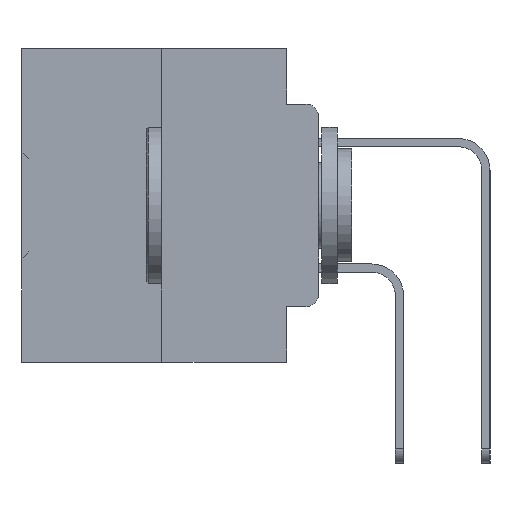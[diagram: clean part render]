
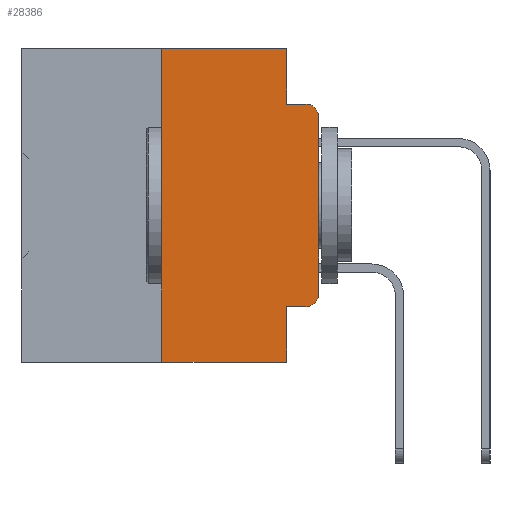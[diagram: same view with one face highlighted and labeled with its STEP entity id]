
A CAD part, left-side view. The second image highlights one B-rep face of the part: STEP entity #28386.
In plain terms, the highlighted planar face has unit normal (-1, 0, 0).
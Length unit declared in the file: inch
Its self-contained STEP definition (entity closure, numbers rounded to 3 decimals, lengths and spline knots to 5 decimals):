
#741 = PLANE ( 'NONE',  #30146 ) ;
#2424 = EDGE_LOOP ( 'NONE', ( #10243, #35201, #12143, #14058, #26782, #34730, #13611, #7345, #28178, #4882 ) ) ;
#2803 = VECTOR ( 'NONE', #15561, 39.37008 ) ;
#3230 = LINE ( 'NONE', #26917, #35577 ) ;
#3666 = DIRECTION ( 'NONE',  ( -1., 0., 0. ) ) ;
#3808 = CARTESIAN_POINT ( 'NONE',  ( 0., 0.02, -0.0885 ) ) ;
#4882 = ORIENTED_EDGE ( 'NONE', *, *, #6563, .T. ) ;
#5681 = CARTESIAN_POINT ( 'NONE',  ( 0., 0.02, -0.4115 ) ) ;
#5981 = CARTESIAN_POINT ( 'NONE',  ( 0., 0., -0.1085 ) ) ;
#6563 = EDGE_CURVE ( 'NONE', #16590, #31774, #32339, .T. ) ;
#6751 = VECTOR ( 'NONE', #33937, 39.37008 ) ;
#7107 = DIRECTION ( 'NONE',  ( 1., 0., 0. ) ) ;
#7345 = ORIENTED_EDGE ( 'NONE', *, *, #12779, .F. ) ;
#7488 = DIRECTION ( 'NONE',  ( -1., 0., 0. ) ) ;
#7568 = LINE ( 'NONE', #31836, #13822 ) ;
#7675 = CIRCLE ( 'NONE', #20356, 0.02 ) ;
#8443 = DIRECTION ( 'NONE',  ( 0., -1., 0. ) ) ;
#8575 = VECTOR ( 'NONE', #8443, 39.37008 ) ;
#8683 = EDGE_CURVE ( 'NONE', #19839, #16590, #31679, .T. ) ;
#8967 = CARTESIAN_POINT ( 'NONE',  ( 0., 0.25, 0. ) ) ;
#10084 = CARTESIAN_POINT ( 'NONE',  ( 0., 0.051, -0.4115 ) ) ;
#10243 = ORIENTED_EDGE ( 'NONE', *, *, #36986, .T. ) ;
#11139 = DIRECTION ( 'NONE',  ( 0., 0., -1. ) ) ;
#11536 = CARTESIAN_POINT ( 'NONE',  ( 0., 0.051, -0.4115 ) ) ;
#12107 = VERTEX_POINT ( 'NONE', #14126 ) ;
#12143 = ORIENTED_EDGE ( 'NONE', *, *, #28910, .F. ) ;
#12469 = CARTESIAN_POINT ( 'NONE',  ( 0., 0.051, -0.0885 ) ) ;
#12779 = EDGE_CURVE ( 'NONE', #19839, #12107, #15942, .T. ) ;
#13611 = ORIENTED_EDGE ( 'NONE', *, *, #34711, .T. ) ;
#13822 = VECTOR ( 'NONE', #16791, 39.37008 ) ;
#14058 = ORIENTED_EDGE ( 'NONE', *, *, #24938, .F. ) ;
#14126 = CARTESIAN_POINT ( 'NONE',  ( 0., 0.051, -0.5 ) ) ;
#14241 = CARTESIAN_POINT ( 'NONE',  ( 0., 0.25, -0.5 ) ) ;
#14665 = VECTOR ( 'NONE', #21084, 39.37008 ) ;
#14982 = VECTOR ( 'NONE', #11139, 39.37008 ) ;
#15395 = VECTOR ( 'NONE', #28337, 39.37008 ) ;
#15561 = DIRECTION ( 'NONE',  ( 0., -1., 0. ) ) ;
#15942 = LINE ( 'NONE', #35222, #14982 ) ;
#16234 = CARTESIAN_POINT ( 'NONE',  ( 0., 0.473, 0. ) ) ;
#16292 = CARTESIAN_POINT ( 'NONE',  ( 0., 0.473, -0.5 ) ) ;
#16363 = VERTEX_POINT ( 'NONE', #25926 ) ;
#16590 = VERTEX_POINT ( 'NONE', #5681 ) ;
#16735 = CARTESIAN_POINT ( 'NONE',  ( 0., 0.051, -0.0885 ) ) ;
#16791 = DIRECTION ( 'NONE',  ( 0., 0., 1. ) ) ;
#19226 = LINE ( 'NONE', #12469, #2803 ) ;
#19839 = VERTEX_POINT ( 'NONE', #10084 ) ;
#20356 = AXIS2_PLACEMENT_3D ( 'NONE', #22087, #3666, #25081 ) ;
#20947 = EDGE_CURVE ( 'NONE', #22070, #16363, #22695, .T. ) ;
#21084 = DIRECTION ( 'NONE',  ( 0., 0., 1. ) ) ;
#21580 = FACE_OUTER_BOUND ( 'NONE', #2424, .T. ) ;
#22070 = VERTEX_POINT ( 'NONE', #14241 ) ;
#22087 = CARTESIAN_POINT ( 'NONE',  ( 0., 0.02, -0.1085 ) ) ;
#22695 = LINE ( 'NONE', #8967, #14665 ) ;
#23668 = AXIS2_PLACEMENT_3D ( 'NONE', #25664, #7488, #28639 ) ;
#23918 = LINE ( 'NONE', #30905, #6751 ) ;
#24938 = EDGE_CURVE ( 'NONE', #38073, #35806, #23918, .T. ) ;
#25081 = DIRECTION ( 'NONE',  ( 0., 0., -1. ) ) ;
#25664 = CARTESIAN_POINT ( 'NONE',  ( 0., 0.02, -0.3915 ) ) ;
#25926 = CARTESIAN_POINT ( 'NONE',  ( 0., 0.25, 0. ) ) ;
#26782 = ORIENTED_EDGE ( 'NONE', *, *, #29525, .F. ) ;
#26917 = CARTESIAN_POINT ( 'NONE',  ( 0., 0.473, 0. ) ) ;
#28178 = ORIENTED_EDGE ( 'NONE', *, *, #8683, .T. ) ;
#28284 = DIRECTION ( 'NONE',  ( 0., 0., -1. ) ) ;
#28337 = DIRECTION ( 'NONE',  ( 0., -1., 0. ) ) ;
#28386 = ADVANCED_FACE ( 'NONE', ( #21580 ), #741, .F. ) ;
#28639 = DIRECTION ( 'NONE',  ( 0., 0., -1. ) ) ;
#28910 = EDGE_CURVE ( 'NONE', #35806, #34992, #19226, .T. ) ;
#29525 = EDGE_CURVE ( 'NONE', #16363, #38073, #3230, .T. ) ;
#30146 = AXIS2_PLACEMENT_3D ( 'NONE', #16234, #7107, #28284 ) ;
#30905 = CARTESIAN_POINT ( 'NONE',  ( 0., 0.051, 0. ) ) ;
#31679 = LINE ( 'NONE', #11536, #8575 ) ;
#31774 = VERTEX_POINT ( 'NONE', #35281 ) ;
#31836 = CARTESIAN_POINT ( 'NONE',  ( 0., 0., 0. ) ) ;
#32273 = LINE ( 'NONE', #16292, #15395 ) ;
#32339 = CIRCLE ( 'NONE', #23668, 0.02 ) ;
#33851 = VERTEX_POINT ( 'NONE', #5981 ) ;
#33937 = DIRECTION ( 'NONE',  ( 0., 0., -1. ) ) ;
#34711 = EDGE_CURVE ( 'NONE', #22070, #12107, #32273, .T. ) ;
#34730 = ORIENTED_EDGE ( 'NONE', *, *, #20947, .F. ) ;
#34950 = EDGE_CURVE ( 'NONE', #33851, #34992, #7675, .T. ) ;
#34992 = VERTEX_POINT ( 'NONE', #3808 ) ;
#35072 = CARTESIAN_POINT ( 'NONE',  ( 0., 0.051, 0. ) ) ;
#35201 = ORIENTED_EDGE ( 'NONE', *, *, #34950, .T. ) ;
#35222 = CARTESIAN_POINT ( 'NONE',  ( 0., 0.051, 0. ) ) ;
#35281 = CARTESIAN_POINT ( 'NONE',  ( 0., 0., -0.3915 ) ) ;
#35577 = VECTOR ( 'NONE', #35975, 39.37008 ) ;
#35806 = VERTEX_POINT ( 'NONE', #16735 ) ;
#35975 = DIRECTION ( 'NONE',  ( 0., -1., 0. ) ) ;
#36986 = EDGE_CURVE ( 'NONE', #31774, #33851, #7568, .T. ) ;
#38073 = VERTEX_POINT ( 'NONE', #35072 ) ;
